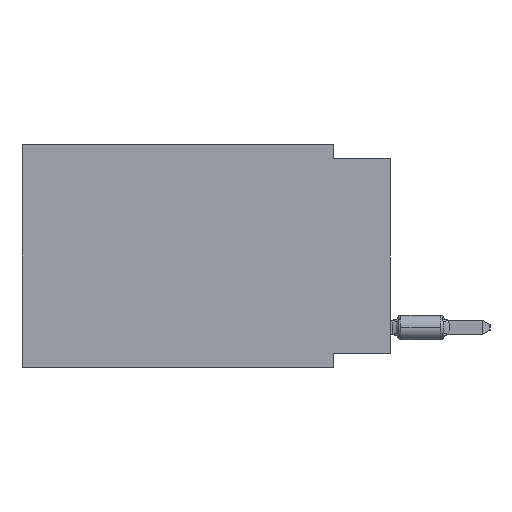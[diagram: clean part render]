
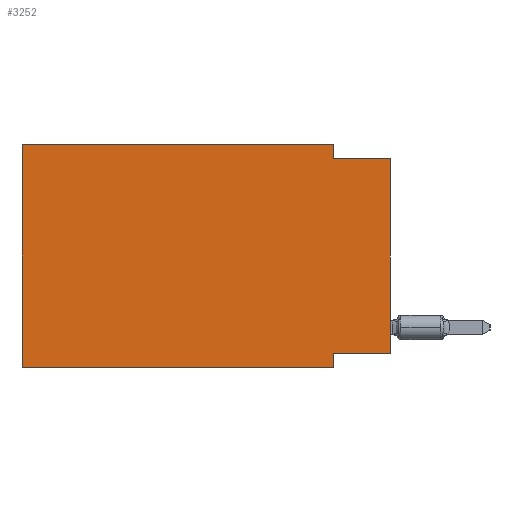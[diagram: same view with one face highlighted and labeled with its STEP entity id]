
A CAD part, left-side view. The second image highlights one B-rep face of the part: STEP entity #3252.
In plain terms, the highlighted planar face has unit normal (-1, 0, 0).
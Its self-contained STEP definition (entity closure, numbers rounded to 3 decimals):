
#44 = CARTESIAN_POINT ( 'NONE',  ( 0., 16.383, -9.906 ) ) ;
#865 = CARTESIAN_POINT ( 'NONE',  ( 0., 16.383, 0. ) ) ;
#1184 = VERTEX_POINT ( 'NONE', #19264 ) ;
#1328 = ORIENTED_EDGE ( 'NONE', *, *, #21416, .F. ) ;
#1594 = VERTEX_POINT ( 'NONE', #1926 ) ;
#1690 = ORIENTED_EDGE ( 'NONE', *, *, #8095, .F. ) ;
#1815 = CARTESIAN_POINT ( 'NONE',  ( 0., 2.54, -9.906 ) ) ;
#1926 = CARTESIAN_POINT ( 'NONE',  ( 0., 2.54, 0. ) ) ;
#2237 = VECTOR ( 'NONE', #11106, 1000. ) ;
#3038 = CARTESIAN_POINT ( 'NONE',  ( 0., 16.383, 0. ) ) ;
#3220 = ORIENTED_EDGE ( 'NONE', *, *, #6067, .F. ) ;
#3252 = ADVANCED_FACE ( 'NONE', ( #12195 ), #17272, .F. ) ;
#3523 = LINE ( 'NONE', #1815, #11390 ) ;
#4131 = CARTESIAN_POINT ( 'NONE',  ( 0., 2.54, -9.271 ) ) ;
#4189 = ORIENTED_EDGE ( 'NONE', *, *, #21856, .T. ) ;
#5038 = VECTOR ( 'NONE', #15757, 1000. ) ;
#5196 = EDGE_CURVE ( 'NONE', #1594, #10438, #14999, .T. ) ;
#5206 = CARTESIAN_POINT ( 'NONE',  ( 0., 2.54, 0. ) ) ;
#5633 = CARTESIAN_POINT ( 'NONE',  ( 0., 16.383, 0. ) ) ;
#6067 = EDGE_CURVE ( 'NONE', #17848, #18620, #17327, .T. ) ;
#6155 = AXIS2_PLACEMENT_3D ( 'NONE', #3038, #11864, #9951 ) ;
#6222 = CARTESIAN_POINT ( 'NONE',  ( 0., 0., -9.271 ) ) ;
#6344 = VECTOR ( 'NONE', #19538, 1000. ) ;
#6895 = DIRECTION ( 'NONE',  ( 0., 0., -1. ) ) ;
#7421 = VECTOR ( 'NONE', #18287, 1000. ) ;
#8095 = EDGE_CURVE ( 'NONE', #10438, #16043, #8929, .T. ) ;
#8891 = EDGE_CURVE ( 'NONE', #17848, #16043, #12799, .T. ) ;
#8929 = LINE ( 'NONE', #13997, #9462 ) ;
#9462 = VECTOR ( 'NONE', #15809, 1000. ) ;
#9598 = LINE ( 'NONE', #5633, #20048 ) ;
#9906 = CARTESIAN_POINT ( 'NONE',  ( 0., 0., -0.635 ) ) ;
#9951 = DIRECTION ( 'NONE',  ( 0., 0., -1. ) ) ;
#10015 = ORIENTED_EDGE ( 'NONE', *, *, #5196, .F. ) ;
#10067 = ORIENTED_EDGE ( 'NONE', *, *, #8891, .T. ) ;
#10438 = VERTEX_POINT ( 'NONE', #11086 ) ;
#10439 = DIRECTION ( 'NONE',  ( 0., 0., -1. ) ) ;
#10789 = CARTESIAN_POINT ( 'NONE',  ( 0., 0., -9.271 ) ) ;
#11086 = CARTESIAN_POINT ( 'NONE',  ( 0., 2.54, -0.635 ) ) ;
#11106 = DIRECTION ( 'NONE',  ( 0., 0., 1. ) ) ;
#11390 = VECTOR ( 'NONE', #10439, 1000. ) ;
#11864 = DIRECTION ( 'NONE',  ( 1., 0., 0. ) ) ;
#12195 = FACE_OUTER_BOUND ( 'NONE', #14392, .T. ) ;
#12799 = LINE ( 'NONE', #12905, #2237 ) ;
#12905 = CARTESIAN_POINT ( 'NONE',  ( 0., 0., 0. ) ) ;
#13309 = VECTOR ( 'NONE', #6895, 1000. ) ;
#13894 = CARTESIAN_POINT ( 'NONE',  ( 0., 16.383, -9.906 ) ) ;
#13997 = CARTESIAN_POINT ( 'NONE',  ( 0., 0., -0.635 ) ) ;
#14119 = VERTEX_POINT ( 'NONE', #20899 ) ;
#14340 = DIRECTION ( 'NONE',  ( 0., -1., 0. ) ) ;
#14392 = EDGE_LOOP ( 'NONE', ( #10067, #1690, #10015, #18967, #20167, #4189, #1328, #3220 ) ) ;
#14999 = LINE ( 'NONE', #5206, #13309 ) ;
#15757 = DIRECTION ( 'NONE',  ( 0., 1., 0. ) ) ;
#15809 = DIRECTION ( 'NONE',  ( 0., -1., 0. ) ) ;
#16043 = VERTEX_POINT ( 'NONE', #9906 ) ;
#16993 = EDGE_CURVE ( 'NONE', #1184, #1594, #9598, .T. ) ;
#17272 = PLANE ( 'NONE',  #6155 ) ;
#17327 = LINE ( 'NONE', #10789, #5038 ) ;
#17848 = VERTEX_POINT ( 'NONE', #6222 ) ;
#18287 = DIRECTION ( 'NONE',  ( 0., 0., 1. ) ) ;
#18620 = VERTEX_POINT ( 'NONE', #4131 ) ;
#18967 = ORIENTED_EDGE ( 'NONE', *, *, #16993, .F. ) ;
#19044 = VERTEX_POINT ( 'NONE', #44 ) ;
#19264 = CARTESIAN_POINT ( 'NONE',  ( 0., 16.383, 0. ) ) ;
#19538 = DIRECTION ( 'NONE',  ( 0., -1., 0. ) ) ;
#20048 = VECTOR ( 'NONE', #14340, 1000. ) ;
#20167 = ORIENTED_EDGE ( 'NONE', *, *, #22059, .F. ) ;
#20899 = CARTESIAN_POINT ( 'NONE',  ( 0., 2.54, -9.906 ) ) ;
#21140 = LINE ( 'NONE', #13894, #6344 ) ;
#21416 = EDGE_CURVE ( 'NONE', #18620, #14119, #3523, .T. ) ;
#21686 = LINE ( 'NONE', #865, #7421 ) ;
#21856 = EDGE_CURVE ( 'NONE', #19044, #14119, #21140, .T. ) ;
#22059 = EDGE_CURVE ( 'NONE', #19044, #1184, #21686, .T. ) ;
